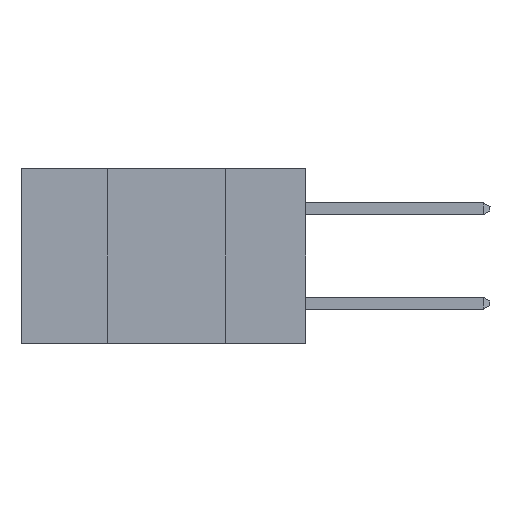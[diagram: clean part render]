
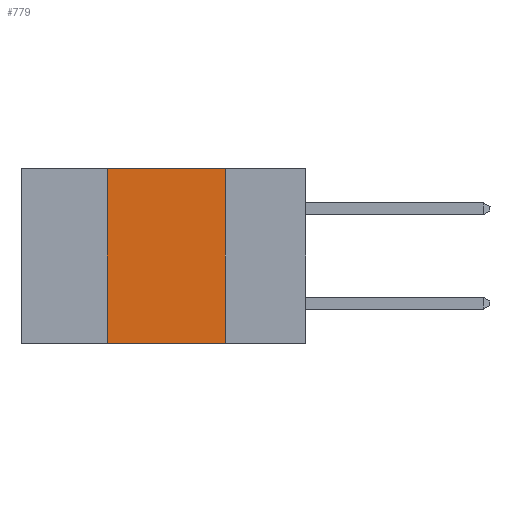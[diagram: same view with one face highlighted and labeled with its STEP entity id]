
A CAD part, left-side view. The second image highlights one B-rep face of the part: STEP entity #779.
In plain terms, the highlighted planar face has unit normal (-1, 0, 0).
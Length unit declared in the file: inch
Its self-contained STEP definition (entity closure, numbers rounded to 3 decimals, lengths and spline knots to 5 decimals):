
#418 = VERTEX_POINT ( 'NONE', #4937 ) ;
#779 = ADVANCED_FACE ( 'NONE', ( #20180 ), #7476, .F. ) ;
#1321 = CARTESIAN_POINT ( 'NONE',  ( 0., 0.6, 0. ) ) ;
#1833 = LINE ( 'NONE', #24893, #18012 ) ;
#2611 = EDGE_CURVE ( 'NONE', #418, #4516, #10741, .T. ) ;
#3238 = CARTESIAN_POINT ( 'NONE',  ( 0., 0.17, 0. ) ) ;
#3960 = VECTOR ( 'NONE', #19390, 39.37008 ) ;
#4061 = ORIENTED_EDGE ( 'NONE', *, *, #9944, .T. ) ;
#4516 = VERTEX_POINT ( 'NONE', #5268 ) ;
#4937 = CARTESIAN_POINT ( 'NONE',  ( 0., 0.42, -0.37 ) ) ;
#5268 = CARTESIAN_POINT ( 'NONE',  ( 0., 0.42, 0. ) ) ;
#5908 = CARTESIAN_POINT ( 'NONE',  ( 0., 0.6, -0.37 ) ) ;
#7476 = PLANE ( 'NONE',  #19715 ) ;
#8602 = ORIENTED_EDGE ( 'NONE', *, *, #17382, .F. ) ;
#8728 = ORIENTED_EDGE ( 'NONE', *, *, #22653, .F. ) ;
#9944 = EDGE_CURVE ( 'NONE', #418, #25961, #13890, .T. ) ;
#10417 = DIRECTION ( 'NONE',  ( 0., -1., 0. ) ) ;
#10741 = LINE ( 'NONE', #15244, #3960 ) ;
#13030 = VECTOR ( 'NONE', #18873, 39.37008 ) ;
#13599 = CARTESIAN_POINT ( 'NONE',  ( 0., 0.17, 0. ) ) ;
#13890 = LINE ( 'NONE', #5908, #16757 ) ;
#15244 = CARTESIAN_POINT ( 'NONE',  ( 0., 0.42, 0. ) ) ;
#16104 = DIRECTION ( 'NONE',  ( 0., -1., 0. ) ) ;
#16584 = CARTESIAN_POINT ( 'NONE',  ( 0., 0.17, -0.37 ) ) ;
#16757 = VECTOR ( 'NONE', #16104, 39.37008 ) ;
#17382 = EDGE_CURVE ( 'NONE', #4516, #21423, #1833, .T. ) ;
#18012 = VECTOR ( 'NONE', #10417, 39.37008 ) ;
#18873 = DIRECTION ( 'NONE',  ( 0., 0., -1. ) ) ;
#19390 = DIRECTION ( 'NONE',  ( 0., 0., 1. ) ) ;
#19715 = AXIS2_PLACEMENT_3D ( 'NONE', #1321, #24084, #21963 ) ;
#20180 = FACE_OUTER_BOUND ( 'NONE', #20686, .T. ) ;
#20686 = EDGE_LOOP ( 'NONE', ( #8728, #8602, #24206, #4061 ) ) ;
#21423 = VERTEX_POINT ( 'NONE', #3238 ) ;
#21963 = DIRECTION ( 'NONE',  ( 0., 0., -1. ) ) ;
#22653 = EDGE_CURVE ( 'NONE', #21423, #25961, #23769, .T. ) ;
#23769 = LINE ( 'NONE', #13599, #13030 ) ;
#24084 = DIRECTION ( 'NONE',  ( 1., 0., 0. ) ) ;
#24206 = ORIENTED_EDGE ( 'NONE', *, *, #2611, .F. ) ;
#24893 = CARTESIAN_POINT ( 'NONE',  ( 0., 0.6, 0. ) ) ;
#25961 = VERTEX_POINT ( 'NONE', #16584 ) ;
